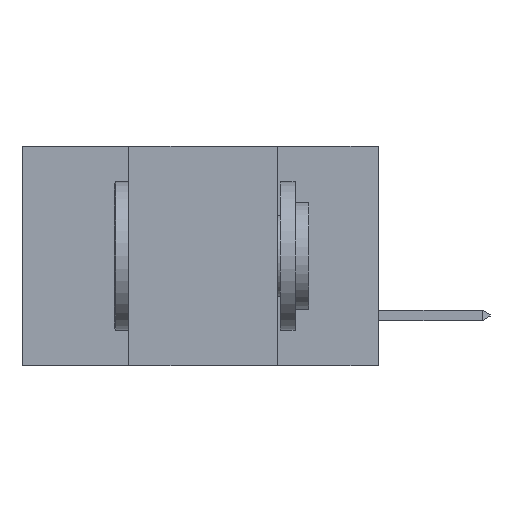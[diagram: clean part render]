
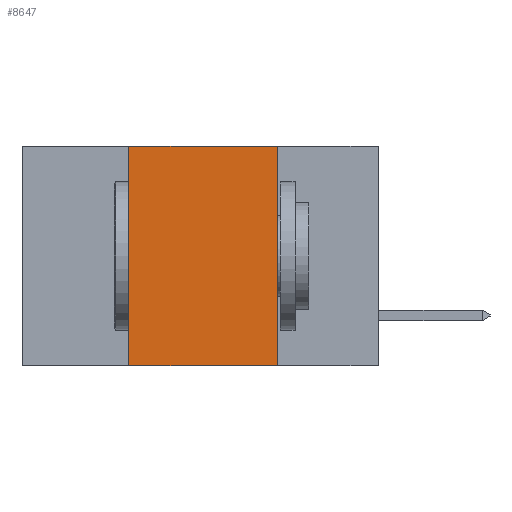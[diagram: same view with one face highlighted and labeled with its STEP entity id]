
A CAD part, left-side view. The second image highlights one B-rep face of the part: STEP entity #8647.
In plain terms, the highlighted planar face has unit normal (-1, 0, 0).
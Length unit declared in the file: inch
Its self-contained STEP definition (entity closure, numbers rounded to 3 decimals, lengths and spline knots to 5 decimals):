
#33 = ORIENTED_EDGE ( 'NONE', *, *, #3900, .T. ) ;
#455 = CARTESIAN_POINT ( 'NONE',  ( 0., 0.17, 0. ) ) ;
#2634 = VERTEX_POINT ( 'NONE', #455 ) ;
#2920 = CARTESIAN_POINT ( 'NONE',  ( 0., 0.6, 0. ) ) ;
#3033 = EDGE_LOOP ( 'NONE', ( #12038, #7525, #3938, #33 ) ) ;
#3480 = VERTEX_POINT ( 'NONE', #11047 ) ;
#3645 = DIRECTION ( 'NONE',  ( 0., 0., -1. ) ) ;
#3900 = EDGE_CURVE ( 'NONE', #4081, #5308, #12740, .T. ) ;
#3930 = DIRECTION ( 'NONE',  ( 0., -1., 0. ) ) ;
#3938 = ORIENTED_EDGE ( 'NONE', *, *, #6234, .F. ) ;
#4004 = CARTESIAN_POINT ( 'NONE',  ( 0., 0.17, 0. ) ) ;
#4081 = VERTEX_POINT ( 'NONE', #20829 ) ;
#5308 = VERTEX_POINT ( 'NONE', #12514 ) ;
#6234 = EDGE_CURVE ( 'NONE', #4081, #3480, #7021, .T. ) ;
#6675 = VECTOR ( 'NONE', #3930, 39.37008 ) ;
#7021 = LINE ( 'NONE', #13704, #10971 ) ;
#7525 = ORIENTED_EDGE ( 'NONE', *, *, #8052, .F. ) ;
#8008 = FACE_OUTER_BOUND ( 'NONE', #3033, .T. ) ;
#8052 = EDGE_CURVE ( 'NONE', #3480, #2634, #15658, .T. ) ;
#8559 = EDGE_CURVE ( 'NONE', #2634, #5308, #14076, .T. ) ;
#8647 = ADVANCED_FACE ( 'NONE', ( #8008 ), #20323, .F. ) ;
#10971 = VECTOR ( 'NONE', #12745, 39.37008 ) ;
#11047 = CARTESIAN_POINT ( 'NONE',  ( 0., 0.42, 0. ) ) ;
#11752 = DIRECTION ( 'NONE',  ( 0., -1., 0. ) ) ;
#12038 = ORIENTED_EDGE ( 'NONE', *, *, #8559, .F. ) ;
#12514 = CARTESIAN_POINT ( 'NONE',  ( 0., 0.17, -0.37 ) ) ;
#12740 = LINE ( 'NONE', #19559, #20936 ) ;
#12745 = DIRECTION ( 'NONE',  ( 0., 0., 1. ) ) ;
#13540 = VECTOR ( 'NONE', #3645, 39.37008 ) ;
#13704 = CARTESIAN_POINT ( 'NONE',  ( 0., 0.42, 0. ) ) ;
#14076 = LINE ( 'NONE', #4004, #13540 ) ;
#15658 = LINE ( 'NONE', #2920, #6675 ) ;
#19559 = CARTESIAN_POINT ( 'NONE',  ( 0., 0.6, -0.37 ) ) ;
#19818 = DIRECTION ( 'NONE',  ( 0., 0., -1. ) ) ;
#20017 = DIRECTION ( 'NONE',  ( 1., 0., 0. ) ) ;
#20179 = CARTESIAN_POINT ( 'NONE',  ( 0., 0.6, 0. ) ) ;
#20323 = PLANE ( 'NONE',  #20362 ) ;
#20362 = AXIS2_PLACEMENT_3D ( 'NONE', #20179, #20017, #19818 ) ;
#20829 = CARTESIAN_POINT ( 'NONE',  ( 0., 0.42, -0.37 ) ) ;
#20936 = VECTOR ( 'NONE', #11752, 39.37008 ) ;
